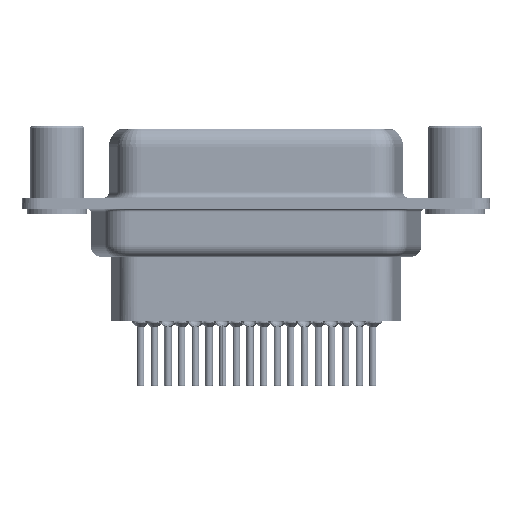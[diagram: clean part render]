
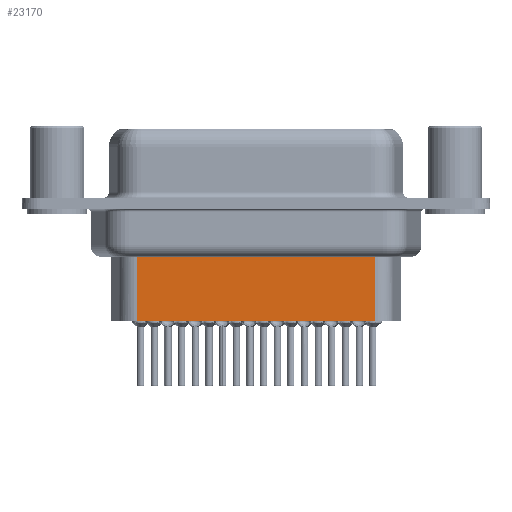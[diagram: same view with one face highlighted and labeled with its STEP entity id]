
A CAD part, front view. The second image highlights one B-rep face of the part: STEP entity #23170.
In plain terms, the highlighted planar face has unit normal (0, -1, 0).
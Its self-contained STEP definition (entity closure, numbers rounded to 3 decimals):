
#328 = VERTEX_POINT ( 'NONE', #19246 ) ;
#781 = AXIS2_PLACEMENT_3D ( 'NONE', #11261, #21565, #31972 ) ;
#1230 = EDGE_CURVE ( 'NONE', #2712, #328, #8252, .T. ) ;
#1667 = LINE ( 'NONE', #2173, #15940 ) ;
#2173 = CARTESIAN_POINT ( 'NONE',  ( 6.691, -3.5, -9.85 ) ) ;
#2712 = VERTEX_POINT ( 'NONE', #12932 ) ;
#4335 = DIRECTION ( 'NONE',  ( 0., 0., -1. ) ) ;
#8252 = LINE ( 'NONE', #14808, #29023 ) ;
#8735 = PLANE ( 'NONE',  #781 ) ;
#11025 = EDGE_CURVE ( 'NONE', #17124, #328, #1667, .T. ) ;
#11261 = CARTESIAN_POINT ( 'NONE',  ( 6.691, -3.5, -3.1 ) ) ;
#12600 = VECTOR ( 'NONE', #17224, 1000. ) ;
#12732 = EDGE_LOOP ( 'NONE', ( #16851, #28993, #21645, #17921 ) ) ;
#12932 = CARTESIAN_POINT ( 'NONE',  ( 6.691, -3.5, -4.097 ) ) ;
#14259 = CARTESIAN_POINT ( 'NONE',  ( 26.629, -3.5, -4.097 ) ) ;
#14808 = CARTESIAN_POINT ( 'NONE',  ( 6.691, -3.5, -3.1 ) ) ;
#15940 = VECTOR ( 'NONE', #33171, 1000. ) ;
#16333 = FACE_OUTER_BOUND ( 'NONE', #12732, .T. ) ;
#16851 = ORIENTED_EDGE ( 'NONE', *, *, #21355, .F. ) ;
#17124 = VERTEX_POINT ( 'NONE', #21541 ) ;
#17224 = DIRECTION ( 'NONE',  ( 0., 0., -1. ) ) ;
#17921 = ORIENTED_EDGE ( 'NONE', *, *, #11025, .F. ) ;
#19246 = CARTESIAN_POINT ( 'NONE',  ( 6.691, -3.5, -9.85 ) ) ;
#19430 = CARTESIAN_POINT ( 'NONE',  ( 26.629, -3.5, -3.1 ) ) ;
#21355 = EDGE_CURVE ( 'NONE', #28509, #17124, #30476, .T. ) ;
#21541 = CARTESIAN_POINT ( 'NONE',  ( 26.629, -3.5, -9.85 ) ) ;
#21565 = DIRECTION ( 'NONE',  ( 0., -1., 0. ) ) ;
#21645 = ORIENTED_EDGE ( 'NONE', *, *, #1230, .T. ) ;
#23170 = ADVANCED_FACE ( 'NONE', ( #16333 ), #8735, .T. ) ;
#24621 = DIRECTION ( 'NONE',  ( -1., 0., 0. ) ) ;
#26440 = EDGE_CURVE ( 'NONE', #28509, #2712, #30070, .T. ) ;
#28509 = VERTEX_POINT ( 'NONE', #14259 ) ;
#28993 = ORIENTED_EDGE ( 'NONE', *, *, #26440, .T. ) ;
#29023 = VECTOR ( 'NONE', #4335, 1000. ) ;
#30070 = LINE ( 'NONE', #32980, #30666 ) ;
#30476 = LINE ( 'NONE', #19430, #12600 ) ;
#30666 = VECTOR ( 'NONE', #24621, 1000. ) ;
#31972 = DIRECTION ( 'NONE',  ( 1., 0., 0. ) ) ;
#32980 = CARTESIAN_POINT ( 'NONE',  ( 6.444, -3.5, -4.097 ) ) ;
#33171 = DIRECTION ( 'NONE',  ( -1., 0., 0. ) ) ;
